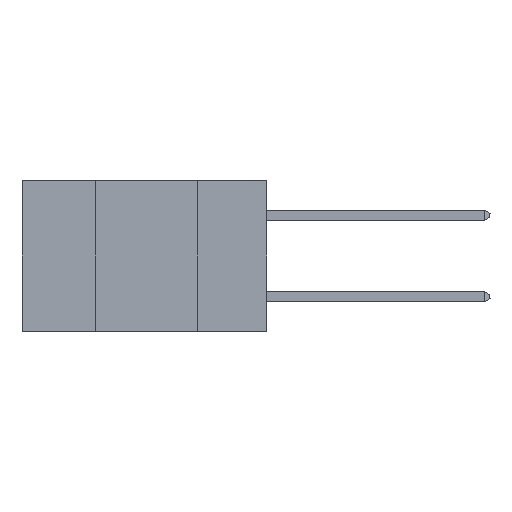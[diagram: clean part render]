
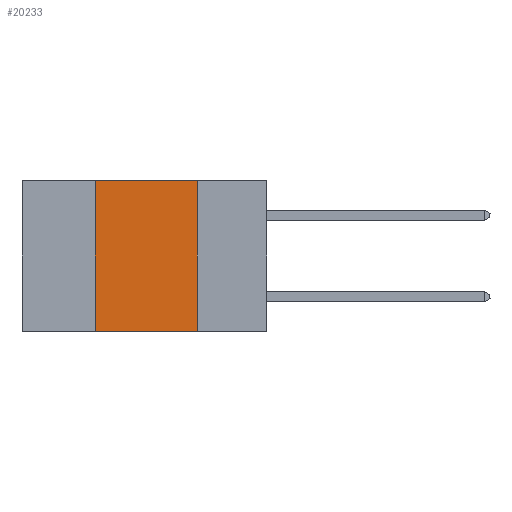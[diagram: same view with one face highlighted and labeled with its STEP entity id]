
A CAD part, left-side view. The second image highlights one B-rep face of the part: STEP entity #20233.
In plain terms, the highlighted planar face has unit normal (-1, 0, 0).
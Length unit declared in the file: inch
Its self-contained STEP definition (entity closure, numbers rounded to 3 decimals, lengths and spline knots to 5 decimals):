
#945 = LINE ( 'NONE', #3098, #18181 ) ;
#2407 = CARTESIAN_POINT ( 'NONE',  ( 0., 0.17, 0. ) ) ;
#2861 = DIRECTION ( 'NONE',  ( 1., 0., 0. ) ) ;
#3098 = CARTESIAN_POINT ( 'NONE',  ( 0., 0.6, -0.37 ) ) ;
#3505 = EDGE_LOOP ( 'NONE', ( #10381, #25593, #16733, #16997 ) ) ;
#3795 = LINE ( 'NONE', #4205, #13247 ) ;
#4205 = CARTESIAN_POINT ( 'NONE',  ( 0., 0.42, 0. ) ) ;
#5453 = DIRECTION ( 'NONE',  ( 0., 0., -1. ) ) ;
#5571 = VECTOR ( 'NONE', #24701, 39.37008 ) ;
#5686 = CARTESIAN_POINT ( 'NONE',  ( 0., 0.42, 0. ) ) ;
#5687 = EDGE_CURVE ( 'NONE', #33310, #7002, #945, .T. ) ;
#6220 = EDGE_CURVE ( 'NONE', #33310, #13855, #3795, .T. ) ;
#7002 = VERTEX_POINT ( 'NONE', #15113 ) ;
#8538 = VECTOR ( 'NONE', #22891, 39.37008 ) ;
#10381 = ORIENTED_EDGE ( 'NONE', *, *, #11287, .F. ) ;
#11235 = CARTESIAN_POINT ( 'NONE',  ( 0., 0.17, 0. ) ) ;
#11287 = EDGE_CURVE ( 'NONE', #18417, #7002, #20330, .T. ) ;
#11771 = DIRECTION ( 'NONE',  ( 0., 0., 1. ) ) ;
#13247 = VECTOR ( 'NONE', #11771, 39.37008 ) ;
#13855 = VERTEX_POINT ( 'NONE', #5686 ) ;
#15113 = CARTESIAN_POINT ( 'NONE',  ( 0., 0.17, -0.37 ) ) ;
#15484 = LINE ( 'NONE', #28133, #8538 ) ;
#16733 = ORIENTED_EDGE ( 'NONE', *, *, #6220, .F. ) ;
#16997 = ORIENTED_EDGE ( 'NONE', *, *, #5687, .T. ) ;
#17201 = AXIS2_PLACEMENT_3D ( 'NONE', #23643, #2861, #5453 ) ;
#18181 = VECTOR ( 'NONE', #29675, 39.37008 ) ;
#18417 = VERTEX_POINT ( 'NONE', #2407 ) ;
#18636 = PLANE ( 'NONE',  #17201 ) ;
#20159 = FACE_OUTER_BOUND ( 'NONE', #3505, .T. ) ;
#20233 = ADVANCED_FACE ( 'NONE', ( #20159 ), #18636, .F. ) ;
#20330 = LINE ( 'NONE', #11235, #5571 ) ;
#22816 = CARTESIAN_POINT ( 'NONE',  ( 0., 0.42, -0.37 ) ) ;
#22891 = DIRECTION ( 'NONE',  ( 0., -1., 0. ) ) ;
#23643 = CARTESIAN_POINT ( 'NONE',  ( 0., 0.6, 0. ) ) ;
#24701 = DIRECTION ( 'NONE',  ( 0., 0., -1. ) ) ;
#25593 = ORIENTED_EDGE ( 'NONE', *, *, #31006, .F. ) ;
#28133 = CARTESIAN_POINT ( 'NONE',  ( 0., 0.6, 0. ) ) ;
#29675 = DIRECTION ( 'NONE',  ( 0., -1., 0. ) ) ;
#31006 = EDGE_CURVE ( 'NONE', #13855, #18417, #15484, .T. ) ;
#33310 = VERTEX_POINT ( 'NONE', #22816 ) ;
